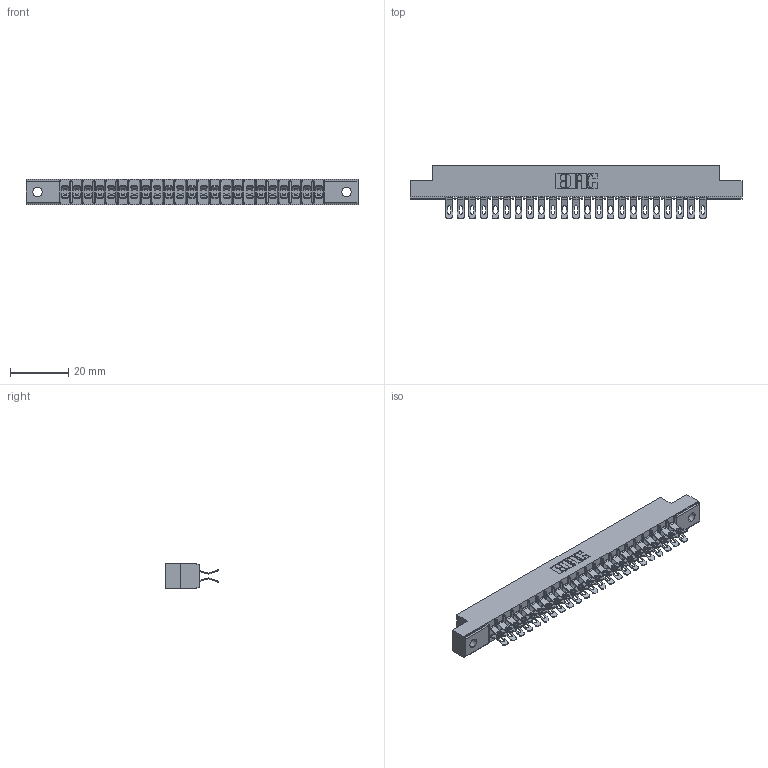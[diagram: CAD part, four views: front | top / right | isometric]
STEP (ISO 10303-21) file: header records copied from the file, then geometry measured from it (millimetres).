
FILE_DESCRIPTION (( 'STEP AP203' ), '1' );
FILE_NAME ('355-046-555-502.STEP', '2019-09-11T14:51:38', ( '' ), ( '' ), 'SwSTEP 2.0', 'SolidWorks 2016', '' );
FILE_SCHEMA (( 'CONFIG_CONTROL_DESIGN' ));
Length unit declared in the file: inch
Products named in the file (3): 305-290-001_555; 305 Part_.128 Dia; 355-046-555-502
Assembly tree (47 placements, depth 2):
  355-046-555-502
    305 Part_.128 Dia
    305-290-001_555  x46
Bounding box: 114.15 x 18.41 x 8.71 mm (x, y, z)
Volume: 6935.5 mm3; surface area: 14400.4 mm2
Topology: 47 solids, 47 shells, 3152 faces, 9401 edges, 6142 vertices
Faces by surface type: plane 1540, cylinder 1520, sphere 92
Entity records: 27842 total; most frequent: CARTESIAN_POINT 4625, ORIENTED_EDGE 4578, DIRECTION 4483, EDGE_CURVE 2289, VECTOR 1811, LINE 1811, VERTEX_POINT 1462, AXIS2_PLACEMENT_3D 1336
